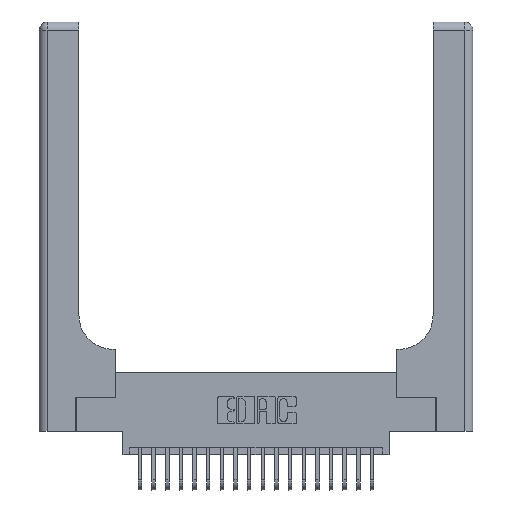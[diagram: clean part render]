
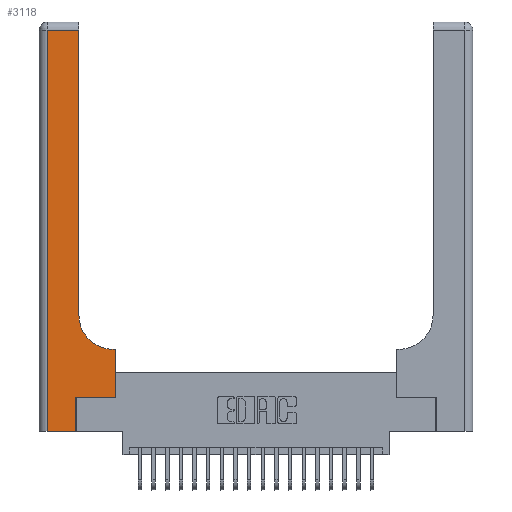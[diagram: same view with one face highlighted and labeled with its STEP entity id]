
A CAD part, top view. The second image highlights one B-rep face of the part: STEP entity #3118.
In plain terms, the highlighted planar face has unit normal (0, 0, 1).
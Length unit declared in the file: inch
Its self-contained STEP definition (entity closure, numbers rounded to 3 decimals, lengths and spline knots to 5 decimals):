
#44 = DIRECTION ( 'NONE',  ( -1., 0., 0. ) ) ;
#420 = CARTESIAN_POINT ( 'NONE',  ( 0.06, 3., 0.37 ) ) ;
#605 = CARTESIAN_POINT ( 'NONE',  ( 0.2915, 0.6, 0.37 ) ) ;
#702 = LINE ( 'NONE', #5163, #13880 ) ;
#918 = VERTEX_POINT ( 'NONE', #15610 ) ;
#1747 = VECTOR ( 'NONE', #13926, 39.37008 ) ;
#1754 = ORIENTED_EDGE ( 'NONE', *, *, #2606, .T. ) ;
#2119 = FACE_OUTER_BOUND ( 'NONE', #12264, .T. ) ;
#2139 = DIRECTION ( 'NONE',  ( 0., -1., 0. ) ) ;
#2212 = CIRCLE ( 'NONE', #21660, 0.25 ) ;
#2230 = CARTESIAN_POINT ( 'NONE',  ( 0.269, 0., 0.37 ) ) ;
#2352 = DIRECTION ( 'NONE',  ( -1., 0., 0. ) ) ;
#2606 = EDGE_CURVE ( 'NONE', #8133, #9248, #2690, .T. ) ;
#2635 = LINE ( 'NONE', #7821, #11782 ) ;
#2690 = LINE ( 'NONE', #8626, #16366 ) ;
#2869 = DIRECTION ( 'NONE',  ( 0., 1., 0. ) ) ;
#3118 = ADVANCED_FACE ( 'NONE', ( #2119 ), #22111, .F. ) ;
#3280 = VECTOR ( 'NONE', #19737, 39.37008 ) ;
#3537 = VECTOR ( 'NONE', #2352, 39.37008 ) ;
#4000 = CARTESIAN_POINT ( 'NONE',  ( 0.269, 0.25, 0.37 ) ) ;
#4050 = EDGE_CURVE ( 'NONE', #8356, #22080, #2635, .T. ) ;
#4435 = VERTEX_POINT ( 'NONE', #2230 ) ;
#4724 = AXIS2_PLACEMENT_3D ( 'NONE', #15336, #20455, #10234 ) ;
#4885 = EDGE_CURVE ( 'NONE', #8798, #8356, #702, .T. ) ;
#5163 = CARTESIAN_POINT ( 'NONE',  ( 0.269, 0.25, 0.37 ) ) ;
#5504 = VERTEX_POINT ( 'NONE', #19535 ) ;
#5971 = EDGE_CURVE ( 'NONE', #18656, #4435, #15460, .T. ) ;
#6804 = DIRECTION ( 'NONE',  ( 1., 0., 0. ) ) ;
#6925 = EDGE_CURVE ( 'NONE', #4435, #8798, #12209, .T. ) ;
#6978 = CARTESIAN_POINT ( 'NONE',  ( 0.5585, 0.6, 0.37 ) ) ;
#7068 = ORIENTED_EDGE ( 'NONE', *, *, #5971, .T. ) ;
#7634 = CARTESIAN_POINT ( 'NONE',  ( 0.2915, 3., 0.37 ) ) ;
#7821 = CARTESIAN_POINT ( 'NONE',  ( 0.5585, 0.25, 0.37 ) ) ;
#7865 = LINE ( 'NONE', #7634, #3280 ) ;
#7984 = CARTESIAN_POINT ( 'NONE',  ( 0.269, 0., 0.37 ) ) ;
#8133 = VERTEX_POINT ( 'NONE', #16306 ) ;
#8134 = EDGE_CURVE ( 'NONE', #918, #8133, #7865, .T. ) ;
#8356 = VERTEX_POINT ( 'NONE', #21650 ) ;
#8626 = CARTESIAN_POINT ( 'NONE',  ( 0., 2.94, 0.37 ) ) ;
#8798 = VERTEX_POINT ( 'NONE', #4000 ) ;
#8939 = ORIENTED_EDGE ( 'NONE', *, *, #4885, .T. ) ;
#9138 = ORIENTED_EDGE ( 'NONE', *, *, #6925, .T. ) ;
#9248 = VERTEX_POINT ( 'NONE', #13782 ) ;
#9323 = CARTESIAN_POINT ( 'NONE',  ( 0.06, 0., 0.37 ) ) ;
#9511 = CARTESIAN_POINT ( 'NONE',  ( 0.5415, 0.85, 0.37 ) ) ;
#10234 = DIRECTION ( 'NONE',  ( -1., 0., 0. ) ) ;
#11258 = DIRECTION ( 'NONE',  ( 1., 0., 0. ) ) ;
#11782 = VECTOR ( 'NONE', #14661, 39.37008 ) ;
#12204 = CARTESIAN_POINT ( 'NONE',  ( 0., 0., 0.37 ) ) ;
#12209 = LINE ( 'NONE', #7984, #16726 ) ;
#12264 = EDGE_LOOP ( 'NONE', ( #16498, #1754, #17597, #7068, #9138, #8939, #13888, #21291, #21983 ) ) ;
#13782 = CARTESIAN_POINT ( 'NONE',  ( 0.06, 2.94, 0.37 ) ) ;
#13880 = VECTOR ( 'NONE', #6804, 39.37008 ) ;
#13888 = ORIENTED_EDGE ( 'NONE', *, *, #4050, .T. ) ;
#13926 = DIRECTION ( 'NONE',  ( 1., 0., 0. ) ) ;
#14661 = DIRECTION ( 'NONE',  ( 0., 1., 0. ) ) ;
#15336 = CARTESIAN_POINT ( 'NONE',  ( 0., 3., 0.37 ) ) ;
#15402 = EDGE_CURVE ( 'NONE', #9248, #18656, #21494, .T. ) ;
#15460 = LINE ( 'NONE', #12204, #1747 ) ;
#15559 = EDGE_CURVE ( 'NONE', #5504, #918, #2212, .T. ) ;
#15610 = CARTESIAN_POINT ( 'NONE',  ( 0.2915, 0.85, 0.37 ) ) ;
#16034 = EDGE_CURVE ( 'NONE', #22080, #5504, #17189, .T. ) ;
#16306 = CARTESIAN_POINT ( 'NONE',  ( 0.2915, 2.94, 0.37 ) ) ;
#16366 = VECTOR ( 'NONE', #44, 39.37008 ) ;
#16498 = ORIENTED_EDGE ( 'NONE', *, *, #8134, .T. ) ;
#16726 = VECTOR ( 'NONE', #2869, 39.37008 ) ;
#17189 = LINE ( 'NONE', #605, #3537 ) ;
#17597 = ORIENTED_EDGE ( 'NONE', *, *, #15402, .T. ) ;
#18656 = VERTEX_POINT ( 'NONE', #9323 ) ;
#19535 = CARTESIAN_POINT ( 'NONE',  ( 0.5415, 0.6, 0.37 ) ) ;
#19737 = DIRECTION ( 'NONE',  ( 0., 1., 0. ) ) ;
#20455 = DIRECTION ( 'NONE',  ( 0., 0., -1. ) ) ;
#20950 = VECTOR ( 'NONE', #2139, 39.37008 ) ;
#21291 = ORIENTED_EDGE ( 'NONE', *, *, #16034, .T. ) ;
#21437 = DIRECTION ( 'NONE',  ( 0., 0., -1. ) ) ;
#21494 = LINE ( 'NONE', #420, #20950 ) ;
#21650 = CARTESIAN_POINT ( 'NONE',  ( 0.5585, 0.25, 0.37 ) ) ;
#21660 = AXIS2_PLACEMENT_3D ( 'NONE', #9511, #21437, #11258 ) ;
#21983 = ORIENTED_EDGE ( 'NONE', *, *, #15559, .T. ) ;
#22080 = VERTEX_POINT ( 'NONE', #6978 ) ;
#22111 = PLANE ( 'NONE',  #4724 ) ;
